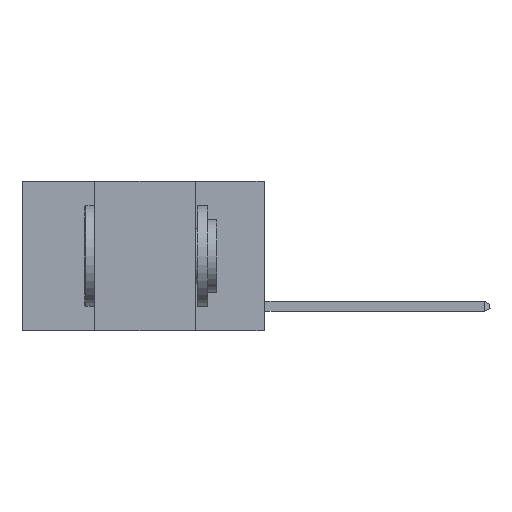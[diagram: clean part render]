
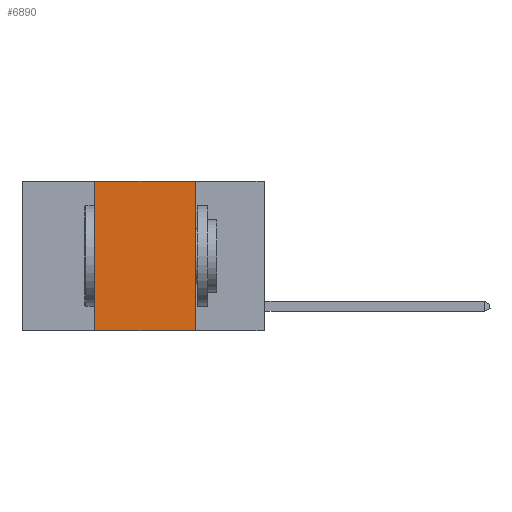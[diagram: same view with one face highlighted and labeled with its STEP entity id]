
A CAD part, left-side view. The second image highlights one B-rep face of the part: STEP entity #6890.
In plain terms, the highlighted planar face has unit normal (-1, 0, 0).
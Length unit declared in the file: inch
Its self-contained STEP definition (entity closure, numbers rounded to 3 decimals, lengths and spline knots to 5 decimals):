
#195 = DIRECTION ( 'NONE',  ( 0., -1., 0. ) ) ;
#360 = LINE ( 'NONE', #6513, #5260 ) ;
#369 = ORIENTED_EDGE ( 'NONE', *, *, #7653, .F. ) ;
#2195 = VERTEX_POINT ( 'NONE', #9571 ) ;
#2455 = CARTESIAN_POINT ( 'NONE',  ( 0., 0.17, 0. ) ) ;
#3057 = EDGE_LOOP ( 'NONE', ( #7835, #369, #11324, #7096 ) ) ;
#3323 = VERTEX_POINT ( 'NONE', #14322 ) ;
#3536 = AXIS2_PLACEMENT_3D ( 'NONE', #6080, #8288, #5774 ) ;
#3787 = LINE ( 'NONE', #2455, #4476 ) ;
#3839 = CARTESIAN_POINT ( 'NONE',  ( 0., 0.17, -0.37 ) ) ;
#4031 = EDGE_CURVE ( 'NONE', #2195, #7060, #360, .T. ) ;
#4476 = VECTOR ( 'NONE', #8633, 39.37008 ) ;
#5260 = VECTOR ( 'NONE', #195, 39.37008 ) ;
#5339 = EDGE_CURVE ( 'NONE', #2195, #3323, #7643, .T. ) ;
#5774 = DIRECTION ( 'NONE',  ( 0., 0., -1. ) ) ;
#6080 = CARTESIAN_POINT ( 'NONE',  ( 0., 0.6, 0. ) ) ;
#6513 = CARTESIAN_POINT ( 'NONE',  ( 0., 0.6, -0.37 ) ) ;
#6890 = ADVANCED_FACE ( 'NONE', ( #10764 ), #9688, .F. ) ;
#7060 = VERTEX_POINT ( 'NONE', #3839 ) ;
#7096 = ORIENTED_EDGE ( 'NONE', *, *, #4031, .T. ) ;
#7111 = CARTESIAN_POINT ( 'NONE',  ( 0., 0.6, 0. ) ) ;
#7236 = CARTESIAN_POINT ( 'NONE',  ( 0., 0.17, 0. ) ) ;
#7643 = LINE ( 'NONE', #9952, #14211 ) ;
#7653 = EDGE_CURVE ( 'NONE', #3323, #8140, #13077, .T. ) ;
#7835 = ORIENTED_EDGE ( 'NONE', *, *, #15447, .F. ) ;
#8140 = VERTEX_POINT ( 'NONE', #7236 ) ;
#8288 = DIRECTION ( 'NONE',  ( 1., 0., 0. ) ) ;
#8633 = DIRECTION ( 'NONE',  ( 0., 0., -1. ) ) ;
#9571 = CARTESIAN_POINT ( 'NONE',  ( 0., 0.42, -0.37 ) ) ;
#9688 = PLANE ( 'NONE',  #3536 ) ;
#9952 = CARTESIAN_POINT ( 'NONE',  ( 0., 0.42, 0. ) ) ;
#10764 = FACE_OUTER_BOUND ( 'NONE', #3057, .T. ) ;
#11324 = ORIENTED_EDGE ( 'NONE', *, *, #5339, .F. ) ;
#12103 = DIRECTION ( 'NONE',  ( 0., -1., 0. ) ) ;
#13077 = LINE ( 'NONE', #7111, #14268 ) ;
#14211 = VECTOR ( 'NONE', #14941, 39.37008 ) ;
#14268 = VECTOR ( 'NONE', #12103, 39.37008 ) ;
#14322 = CARTESIAN_POINT ( 'NONE',  ( 0., 0.42, 0. ) ) ;
#14941 = DIRECTION ( 'NONE',  ( 0., 0., 1. ) ) ;
#15447 = EDGE_CURVE ( 'NONE', #8140, #7060, #3787, .T. ) ;
